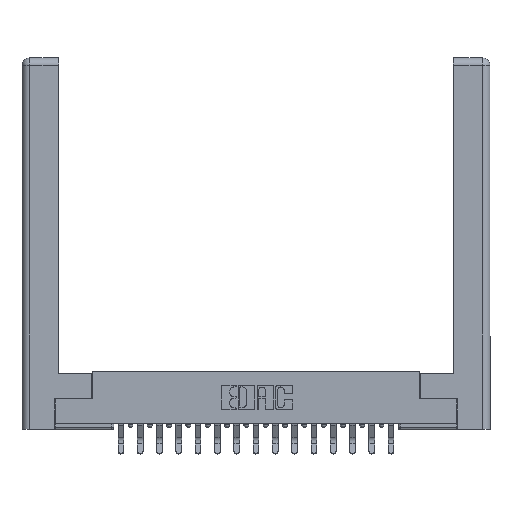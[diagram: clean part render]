
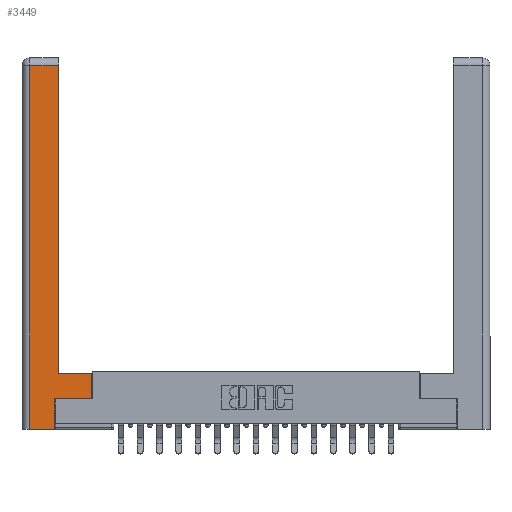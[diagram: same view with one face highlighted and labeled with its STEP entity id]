
A CAD part, top view. The second image highlights one B-rep face of the part: STEP entity #3449.
In plain terms, the highlighted planar face has unit normal (0, 0, 1).
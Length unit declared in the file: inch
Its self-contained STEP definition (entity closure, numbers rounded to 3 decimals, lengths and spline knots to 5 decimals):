
#145 = VERTEX_POINT ( 'NONE', #18381 ) ;
#381 = CARTESIAN_POINT ( 'NONE',  ( 0.295, 0.45, 0. ) ) ;
#838 = ORIENTED_EDGE ( 'NONE', *, *, #16766, .T. ) ;
#1229 = EDGE_CURVE ( 'NONE', #17153, #16268, #3883, .T. ) ;
#1447 = EDGE_LOOP ( 'NONE', ( #6936, #6366, #838, #19265, #10413, #3561, #10861, #17897 ) ) ;
#2169 = CARTESIAN_POINT ( 'NONE',  ( 0.265, 0.245, 0. ) ) ;
#2312 = VECTOR ( 'NONE', #16351, 39.37008 ) ;
#2909 = CARTESIAN_POINT ( 'NONE',  ( 0., 0., 0. ) ) ;
#3449 = ADVANCED_FACE ( 'NONE', ( #6428 ), #11906, .F. ) ;
#3474 = LINE ( 'NONE', #17919, #2312 ) ;
#3561 = ORIENTED_EDGE ( 'NONE', *, *, #10541, .T. ) ;
#3883 = LINE ( 'NONE', #14889, #9985 ) ;
#4171 = CARTESIAN_POINT ( 'NONE',  ( 0.265, 0., 0. ) ) ;
#4250 = VECTOR ( 'NONE', #17334, 39.37008 ) ;
#4770 = DIRECTION ( 'NONE',  ( 0., 0., -1. ) ) ;
#5911 = DIRECTION ( 'NONE',  ( 0., 1., 0. ) ) ;
#6232 = EDGE_CURVE ( 'NONE', #6930, #11006, #16024, .T. ) ;
#6284 = DIRECTION ( 'NONE',  ( -1., 0., 0. ) ) ;
#6366 = ORIENTED_EDGE ( 'NONE', *, *, #6232, .T. ) ;
#6428 = FACE_OUTER_BOUND ( 'NONE', #1447, .T. ) ;
#6613 = CARTESIAN_POINT ( 'NONE',  ( 0.565, 0.245, 0. ) ) ;
#6902 = AXIS2_PLACEMENT_3D ( 'NONE', #2909, #4770, #15591 ) ;
#6930 = VERTEX_POINT ( 'NONE', #10933 ) ;
#6936 = ORIENTED_EDGE ( 'NONE', *, *, #13514, .T. ) ;
#8371 = VECTOR ( 'NONE', #12392, 39.37008 ) ;
#9321 = LINE ( 'NONE', #16125, #11001 ) ;
#9465 = VECTOR ( 'NONE', #18249, 39.37008 ) ;
#9985 = VECTOR ( 'NONE', #5911, 39.37008 ) ;
#10181 = VECTOR ( 'NONE', #6284, 39.37008 ) ;
#10413 = ORIENTED_EDGE ( 'NONE', *, *, #17171, .T. ) ;
#10541 = EDGE_CURVE ( 'NONE', #145, #17153, #19383, .T. ) ;
#10838 = LINE ( 'NONE', #11489, #4250 ) ;
#10861 = ORIENTED_EDGE ( 'NONE', *, *, #1229, .T. ) ;
#10933 = CARTESIAN_POINT ( 'NONE',  ( 0.295, 2.94, 0. ) ) ;
#10960 = CARTESIAN_POINT ( 'NONE',  ( 0.565, 0.245, 0. ) ) ;
#11001 = VECTOR ( 'NONE', #14483, 39.37008 ) ;
#11006 = VERTEX_POINT ( 'NONE', #17929 ) ;
#11489 = CARTESIAN_POINT ( 'NONE',  ( 0.295, 0.45, 0. ) ) ;
#11906 = PLANE ( 'NONE',  #6902 ) ;
#12392 = DIRECTION ( 'NONE',  ( 1., 0., 0. ) ) ;
#12488 = VERTEX_POINT ( 'NONE', #381 ) ;
#12534 = DIRECTION ( 'NONE',  ( 0., 1., 0. ) ) ;
#12612 = VECTOR ( 'NONE', #12534, 39.37008 ) ;
#12838 = VERTEX_POINT ( 'NONE', #4171 ) ;
#13514 = EDGE_CURVE ( 'NONE', #12488, #6930, #13926, .T. ) ;
#13593 = VERTEX_POINT ( 'NONE', #18059 ) ;
#13795 = CARTESIAN_POINT ( 'NONE',  ( 0.295, 3., 0. ) ) ;
#13926 = LINE ( 'NONE', #13795, #9465 ) ;
#14483 = DIRECTION ( 'NONE',  ( 0., -1., 0. ) ) ;
#14541 = EDGE_CURVE ( 'NONE', #16268, #12488, #10838, .T. ) ;
#14889 = CARTESIAN_POINT ( 'NONE',  ( 0.565, 0.45, 0. ) ) ;
#15591 = DIRECTION ( 'NONE',  ( -1., 0., 0. ) ) ;
#15787 = CARTESIAN_POINT ( 'NONE',  ( 0.565, 0.45, 0. ) ) ;
#16024 = LINE ( 'NONE', #18398, #10181 ) ;
#16125 = CARTESIAN_POINT ( 'NONE',  ( 0.0615, 0., 0. ) ) ;
#16268 = VERTEX_POINT ( 'NONE', #15787 ) ;
#16351 = DIRECTION ( 'NONE',  ( 1., 0., 0. ) ) ;
#16584 = LINE ( 'NONE', #2169, #12612 ) ;
#16766 = EDGE_CURVE ( 'NONE', #11006, #13593, #9321, .T. ) ;
#17153 = VERTEX_POINT ( 'NONE', #6613 ) ;
#17171 = EDGE_CURVE ( 'NONE', #12838, #145, #16584, .T. ) ;
#17334 = DIRECTION ( 'NONE',  ( -1., 0., 0. ) ) ;
#17897 = ORIENTED_EDGE ( 'NONE', *, *, #14541, .T. ) ;
#17919 = CARTESIAN_POINT ( 'NONE',  ( 0.265, 0., 0. ) ) ;
#17929 = CARTESIAN_POINT ( 'NONE',  ( 0.0615, 2.94, 0. ) ) ;
#18059 = CARTESIAN_POINT ( 'NONE',  ( 0.0615, 0., 0. ) ) ;
#18078 = EDGE_CURVE ( 'NONE', #13593, #12838, #3474, .T. ) ;
#18249 = DIRECTION ( 'NONE',  ( 0., 1., 0. ) ) ;
#18381 = CARTESIAN_POINT ( 'NONE',  ( 0.265, 0.245, 0. ) ) ;
#18398 = CARTESIAN_POINT ( 'NONE',  ( 0.0615, 2.94, 0. ) ) ;
#19265 = ORIENTED_EDGE ( 'NONE', *, *, #18078, .T. ) ;
#19383 = LINE ( 'NONE', #10960, #8371 ) ;
